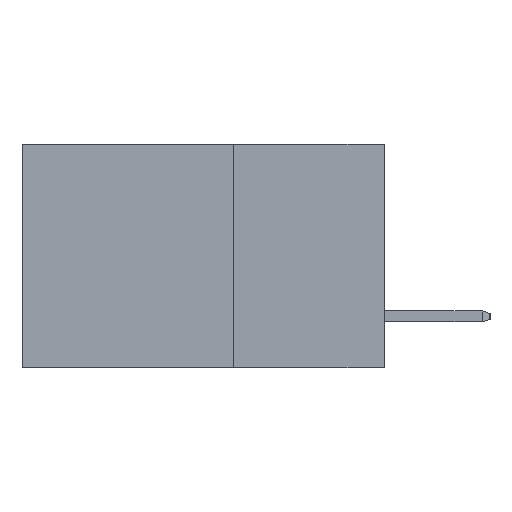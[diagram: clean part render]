
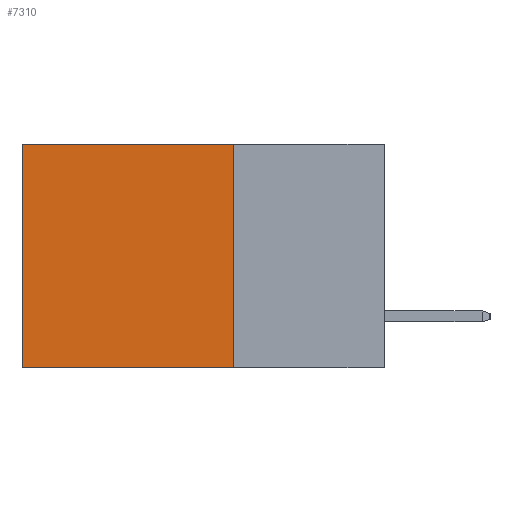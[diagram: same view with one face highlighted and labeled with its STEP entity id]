
A CAD part, left-side view. The second image highlights one B-rep face of the part: STEP entity #7310.
In plain terms, the highlighted planar face has unit normal (-1, 0, 0).
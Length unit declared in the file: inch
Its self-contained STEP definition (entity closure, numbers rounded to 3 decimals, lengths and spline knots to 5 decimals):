
#181 = CARTESIAN_POINT ( 'NONE',  ( 0.2615, 0.25, 0. ) ) ;
#672 = ORIENTED_EDGE ( 'NONE', *, *, #4037, .T. ) ;
#906 = LINE ( 'NONE', #6640, #10925 ) ;
#1118 = CARTESIAN_POINT ( 'NONE',  ( 0.2615, 0.25, -0.37 ) ) ;
#1160 = ORIENTED_EDGE ( 'NONE', *, *, #2224, .F. ) ;
#2021 = ORIENTED_EDGE ( 'NONE', *, *, #2127, .T. ) ;
#2127 = EDGE_CURVE ( 'NONE', #9200, #4452, #6620, .T. ) ;
#2224 = EDGE_CURVE ( 'NONE', #9526, #9795, #5407, .T. ) ;
#2478 = EDGE_LOOP ( 'NONE', ( #2021, #8856, #1160, #672 ) ) ;
#2765 = DIRECTION ( 'NONE',  ( 0., 1., 0. ) ) ;
#3611 = CARTESIAN_POINT ( 'NONE',  ( 0.2615, 0.25, -0.37 ) ) ;
#4037 = EDGE_CURVE ( 'NONE', #9526, #9200, #9621, .T. ) ;
#4452 = VERTEX_POINT ( 'NONE', #10361 ) ;
#5029 = CARTESIAN_POINT ( 'NONE',  ( 0.2615, 0.6, -0.37 ) ) ;
#5098 = CARTESIAN_POINT ( 'NONE',  ( 0.2615, 0.25, 0. ) ) ;
#5407 = LINE ( 'NONE', #1118, #7981 ) ;
#5536 = CARTESIAN_POINT ( 'NONE',  ( 0.2615, 0.6, 0. ) ) ;
#6402 = DIRECTION ( 'NONE',  ( 0., 1., 0. ) ) ;
#6620 = LINE ( 'NONE', #5029, #11701 ) ;
#6640 = CARTESIAN_POINT ( 'NONE',  ( 0.2615, 0.25, -0.37 ) ) ;
#7047 = VECTOR ( 'NONE', #6402, 39.37008 ) ;
#7310 = ADVANCED_FACE ( 'NONE', ( #9552 ), #8071, .F. ) ;
#7977 = DIRECTION ( 'NONE',  ( 0., 0., -1. ) ) ;
#7981 = VECTOR ( 'NONE', #10621, 39.37008 ) ;
#7994 = DIRECTION ( 'NONE',  ( 1., 0., 0. ) ) ;
#8071 = PLANE ( 'NONE',  #10942 ) ;
#8102 = CARTESIAN_POINT ( 'NONE',  ( 0.2615, 0.25, -0.37 ) ) ;
#8856 = ORIENTED_EDGE ( 'NONE', *, *, #11460, .F. ) ;
#9200 = VERTEX_POINT ( 'NONE', #5536 ) ;
#9526 = VERTEX_POINT ( 'NONE', #181 ) ;
#9552 = FACE_OUTER_BOUND ( 'NONE', #2478, .T. ) ;
#9621 = LINE ( 'NONE', #5098, #7047 ) ;
#9795 = VERTEX_POINT ( 'NONE', #3611 ) ;
#10063 = DIRECTION ( 'NONE',  ( 0., 0., -1. ) ) ;
#10361 = CARTESIAN_POINT ( 'NONE',  ( 0.2615, 0.6, -0.37 ) ) ;
#10621 = DIRECTION ( 'NONE',  ( 0., 0., -1. ) ) ;
#10925 = VECTOR ( 'NONE', #2765, 39.37008 ) ;
#10942 = AXIS2_PLACEMENT_3D ( 'NONE', #8102, #7994, #7977 ) ;
#11460 = EDGE_CURVE ( 'NONE', #9795, #4452, #906, .T. ) ;
#11701 = VECTOR ( 'NONE', #10063, 39.37008 ) ;
